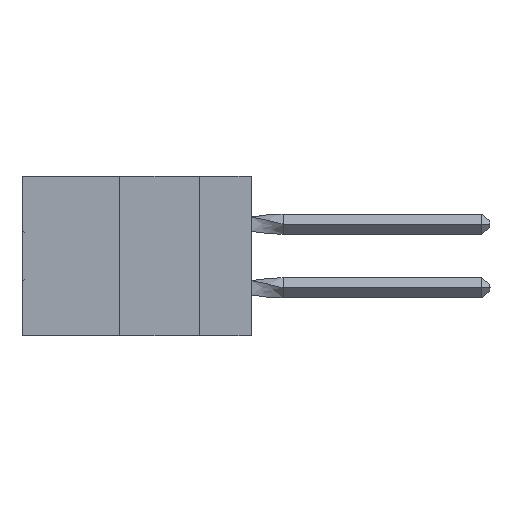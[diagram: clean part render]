
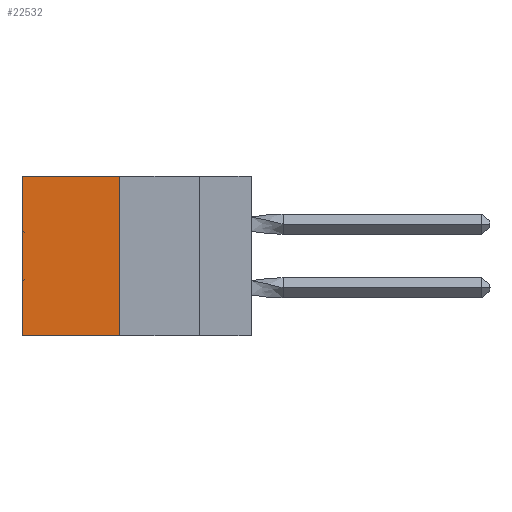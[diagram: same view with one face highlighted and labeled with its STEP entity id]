
A CAD part, left-side view. The second image highlights one B-rep face of the part: STEP entity #22532.
In plain terms, the highlighted planar face has unit normal (-1, 0, 0).
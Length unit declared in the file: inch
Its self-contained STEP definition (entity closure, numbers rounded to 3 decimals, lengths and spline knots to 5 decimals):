
#500 = EDGE_LOOP ( 'NONE', ( #24251, #31362, #28344, #15975 ) ) ;
#2496 = VECTOR ( 'NONE', #12593, 39.37008 ) ;
#3659 = CARTESIAN_POINT ( 'NONE',  ( 0.305, 0.413, -0.5 ) ) ;
#4671 = CARTESIAN_POINT ( 'NONE',  ( 0.305, 0.413, -0.5 ) ) ;
#8435 = VERTEX_POINT ( 'NONE', #10365 ) ;
#10365 = CARTESIAN_POINT ( 'NONE',  ( 0.305, 0.72, -0.5 ) ) ;
#11355 = VERTEX_POINT ( 'NONE', #44557 ) ;
#12593 = DIRECTION ( 'NONE',  ( 0., 0., -1. ) ) ;
#12879 = CARTESIAN_POINT ( 'NONE',  ( 0.305, 0.413, 0. ) ) ;
#14671 = FACE_OUTER_BOUND ( 'NONE', #500, .T. ) ;
#15975 = ORIENTED_EDGE ( 'NONE', *, *, #16025, .T. ) ;
#16025 = EDGE_CURVE ( 'NONE', #11355, #20164, #18976, .T. ) ;
#17326 = DIRECTION ( 'NONE',  ( 0., 0., -1. ) ) ;
#17329 = DIRECTION ( 'NONE',  ( 1., 0., 0. ) ) ;
#18976 = LINE ( 'NONE', #12879, #37156 ) ;
#20164 = VERTEX_POINT ( 'NONE', #32851 ) ;
#21008 = EDGE_CURVE ( 'NONE', #23862, #8435, #50595, .T. ) ;
#21255 = DIRECTION ( 'NONE',  ( 0., 1., 0. ) ) ;
#22532 = ADVANCED_FACE ( 'NONE', ( #14671 ), #42259, .F. ) ;
#23745 = EDGE_CURVE ( 'NONE', #11355, #23862, #50948, .T. ) ;
#23862 = VERTEX_POINT ( 'NONE', #3659 ) ;
#24251 = ORIENTED_EDGE ( 'NONE', *, *, #24573, .T. ) ;
#24573 = EDGE_CURVE ( 'NONE', #20164, #8435, #36453, .T. ) ;
#28344 = ORIENTED_EDGE ( 'NONE', *, *, #23745, .F. ) ;
#31362 = ORIENTED_EDGE ( 'NONE', *, *, #21008, .F. ) ;
#31707 = CARTESIAN_POINT ( 'NONE',  ( 0.305, 0.413, -0.5 ) ) ;
#32628 = VECTOR ( 'NONE', #17326, 39.37008 ) ;
#32851 = CARTESIAN_POINT ( 'NONE',  ( 0.305, 0.72, 0. ) ) ;
#36453 = LINE ( 'NONE', #41877, #2496 ) ;
#36838 = VECTOR ( 'NONE', #52717, 39.37008 ) ;
#37156 = VECTOR ( 'NONE', #21255, 39.37008 ) ;
#41877 = CARTESIAN_POINT ( 'NONE',  ( 0.305, 0.72, -0.5 ) ) ;
#42257 = CARTESIAN_POINT ( 'NONE',  ( 0.305, 0.413, -0.5 ) ) ;
#42259 = PLANE ( 'NONE',  #50114 ) ;
#44557 = CARTESIAN_POINT ( 'NONE',  ( 0.305, 0.413, 0. ) ) ;
#46482 = DIRECTION ( 'NONE',  ( 0., 0., -1. ) ) ;
#50114 = AXIS2_PLACEMENT_3D ( 'NONE', #4671, #17329, #46482 ) ;
#50595 = LINE ( 'NONE', #31707, #36838 ) ;
#50948 = LINE ( 'NONE', #42257, #32628 ) ;
#52717 = DIRECTION ( 'NONE',  ( 0., 1., 0. ) ) ;
